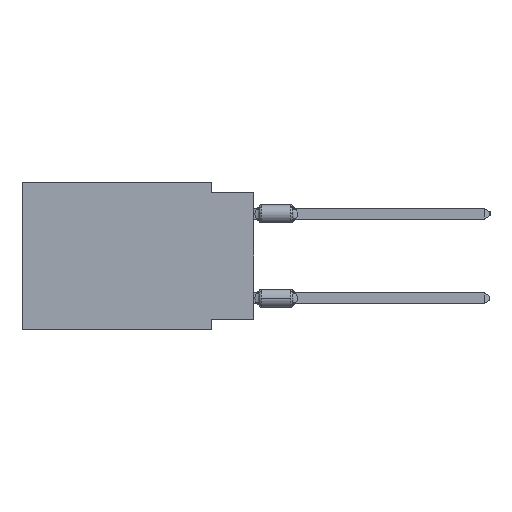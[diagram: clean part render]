
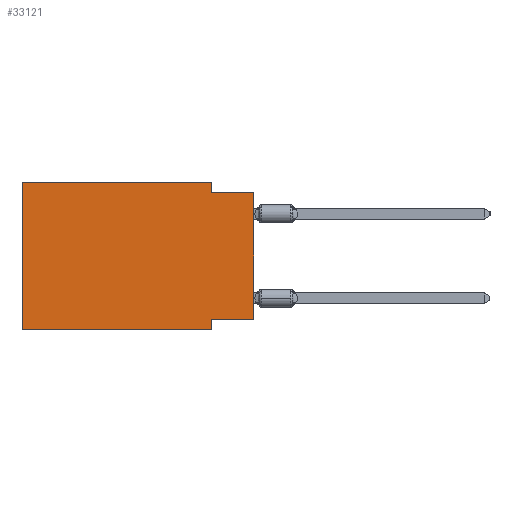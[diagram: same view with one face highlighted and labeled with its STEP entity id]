
A CAD part, left-side view. The second image highlights one B-rep face of the part: STEP entity #33121.
In plain terms, the highlighted planar face has unit normal (-1, 0, 0).
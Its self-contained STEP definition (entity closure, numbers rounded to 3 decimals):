
#1089 = LINE ( 'NONE', #2351, #23914 ) ;
#1787 = LINE ( 'NONE', #48260, #4649 ) ;
#2117 = DIRECTION ( 'NONE',  ( 0., 0., -1. ) ) ;
#2351 = CARTESIAN_POINT ( 'NONE',  ( 0., 0., -0.635 ) ) ;
#3954 = VERTEX_POINT ( 'NONE', #14087 ) ;
#4058 = VERTEX_POINT ( 'NONE', #43259 ) ;
#4649 = VECTOR ( 'NONE', #36645, 1000. ) ;
#4660 = LINE ( 'NONE', #20050, #30097 ) ;
#5016 = VECTOR ( 'NONE', #43256, 1000. ) ;
#6075 = CARTESIAN_POINT ( 'NONE',  ( 0., 2.54, 0. ) ) ;
#6519 = EDGE_LOOP ( 'NONE', ( #23653, #25829, #8789, #17534, #36767, #10336, #32234, #15648 ) ) ;
#7685 = DIRECTION ( 'NONE',  ( 0., 0., 1. ) ) ;
#8097 = DIRECTION ( 'NONE',  ( 0., -1., 0. ) ) ;
#8789 = ORIENTED_EDGE ( 'NONE', *, *, #17099, .F. ) ;
#9693 = VERTEX_POINT ( 'NONE', #17144 ) ;
#10336 = ORIENTED_EDGE ( 'NONE', *, *, #21393, .T. ) ;
#10480 = EDGE_CURVE ( 'NONE', #45519, #41169, #1787, .T. ) ;
#11389 = VERTEX_POINT ( 'NONE', #22799 ) ;
#14087 = CARTESIAN_POINT ( 'NONE',  ( 0., 13.97, -8.89 ) ) ;
#14629 = LINE ( 'NONE', #30037, #5016 ) ;
#15208 = VERTEX_POINT ( 'NONE', #37182 ) ;
#15648 = ORIENTED_EDGE ( 'NONE', *, *, #32006, .F. ) ;
#17099 = EDGE_CURVE ( 'NONE', #35390, #4058, #31086, .T. ) ;
#17144 = CARTESIAN_POINT ( 'NONE',  ( 0., 2.54, -8.255 ) ) ;
#17534 = ORIENTED_EDGE ( 'NONE', *, *, #21677, .F. ) ;
#18952 = VECTOR ( 'NONE', #7685, 1000. ) ;
#19068 = PLANE ( 'NONE',  #38055 ) ;
#19666 = CARTESIAN_POINT ( 'NONE',  ( 0., 0., -0.635 ) ) ;
#20050 = CARTESIAN_POINT ( 'NONE',  ( 0., 0., -8.255 ) ) ;
#21393 = EDGE_CURVE ( 'NONE', #3954, #15208, #35108, .T. ) ;
#21569 = CARTESIAN_POINT ( 'NONE',  ( 0., 2.54, -8.89 ) ) ;
#21677 = EDGE_CURVE ( 'NONE', #11389, #35390, #14629, .T. ) ;
#22799 = CARTESIAN_POINT ( 'NONE',  ( 0., 13.97, 0. ) ) ;
#22923 = EDGE_CURVE ( 'NONE', #4058, #41169, #1089, .T. ) ;
#23104 = DIRECTION ( 'NONE',  ( 0., 1., 0. ) ) ;
#23653 = ORIENTED_EDGE ( 'NONE', *, *, #10480, .T. ) ;
#23914 = VECTOR ( 'NONE', #29379, 1000. ) ;
#25082 = LINE ( 'NONE', #21569, #40518 ) ;
#25829 = ORIENTED_EDGE ( 'NONE', *, *, #22923, .F. ) ;
#27525 = DIRECTION ( 'NONE',  ( 0., 0., -1. ) ) ;
#29379 = DIRECTION ( 'NONE',  ( 0., -1., 0. ) ) ;
#29669 = EDGE_CURVE ( 'NONE', #9693, #15208, #25082, .T. ) ;
#30037 = CARTESIAN_POINT ( 'NONE',  ( 0., 13.97, 0. ) ) ;
#30097 = VECTOR ( 'NONE', #23104, 1000. ) ;
#31086 = LINE ( 'NONE', #46219, #42194 ) ;
#32006 = EDGE_CURVE ( 'NONE', #45519, #9693, #4660, .T. ) ;
#32234 = ORIENTED_EDGE ( 'NONE', *, *, #29669, .F. ) ;
#33121 = ADVANCED_FACE ( 'NONE', ( #49136 ), #19068, .F. ) ;
#33448 = VECTOR ( 'NONE', #8097, 1000. ) ;
#34469 = CARTESIAN_POINT ( 'NONE',  ( 0., 13.97, 0. ) ) ;
#34676 = CARTESIAN_POINT ( 'NONE',  ( 0., 13.97, 0. ) ) ;
#35108 = LINE ( 'NONE', #38162, #33448 ) ;
#35390 = VERTEX_POINT ( 'NONE', #6075 ) ;
#36645 = DIRECTION ( 'NONE',  ( 0., 0., 1. ) ) ;
#36767 = ORIENTED_EDGE ( 'NONE', *, *, #49611, .F. ) ;
#37182 = CARTESIAN_POINT ( 'NONE',  ( 0., 2.54, -8.89 ) ) ;
#37246 = DIRECTION ( 'NONE',  ( 0., 0., -1. ) ) ;
#38055 = AXIS2_PLACEMENT_3D ( 'NONE', #34469, #48896, #37246 ) ;
#38162 = CARTESIAN_POINT ( 'NONE',  ( 0., 13.97, -8.89 ) ) ;
#40518 = VECTOR ( 'NONE', #2117, 1000. ) ;
#41055 = CARTESIAN_POINT ( 'NONE',  ( 0., 0., -8.255 ) ) ;
#41169 = VERTEX_POINT ( 'NONE', #19666 ) ;
#41274 = LINE ( 'NONE', #34676, #18952 ) ;
#42194 = VECTOR ( 'NONE', #27525, 1000. ) ;
#43256 = DIRECTION ( 'NONE',  ( 0., -1., 0. ) ) ;
#43259 = CARTESIAN_POINT ( 'NONE',  ( 0., 2.54, -0.635 ) ) ;
#45519 = VERTEX_POINT ( 'NONE', #41055 ) ;
#46219 = CARTESIAN_POINT ( 'NONE',  ( 0., 2.54, 0. ) ) ;
#48260 = CARTESIAN_POINT ( 'NONE',  ( 0., 0., 0. ) ) ;
#48896 = DIRECTION ( 'NONE',  ( 1., 0., 0. ) ) ;
#49136 = FACE_OUTER_BOUND ( 'NONE', #6519, .T. ) ;
#49611 = EDGE_CURVE ( 'NONE', #3954, #11389, #41274, .T. ) ;
